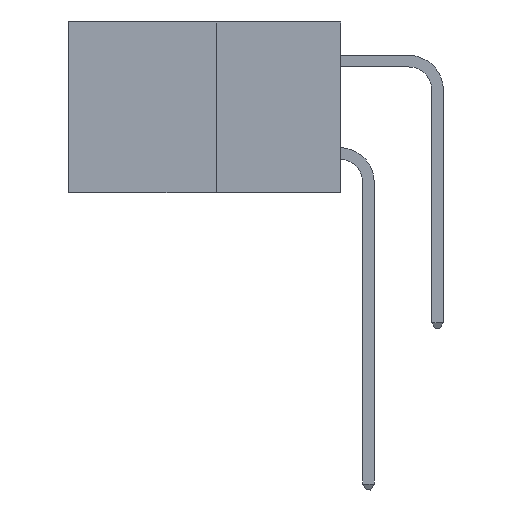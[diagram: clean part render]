
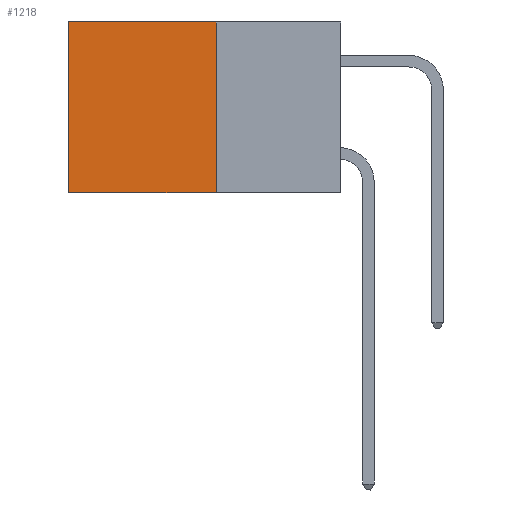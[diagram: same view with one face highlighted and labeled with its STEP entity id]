
A CAD part, left-side view. The second image highlights one B-rep face of the part: STEP entity #1218.
In plain terms, the highlighted planar face has unit normal (-1, 0, 0).
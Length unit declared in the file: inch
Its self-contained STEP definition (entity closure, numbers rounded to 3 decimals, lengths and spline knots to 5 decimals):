
#295 = VERTEX_POINT ( 'NONE', #11340 ) ;
#1195 = DIRECTION ( 'NONE',  ( 0., 0., -1. ) ) ;
#1201 = LINE ( 'NONE', #16741, #13719 ) ;
#1218 = ADVANCED_FACE ( 'NONE', ( #13473 ), #5153, .F. ) ;
#2496 = ORIENTED_EDGE ( 'NONE', *, *, #3451, .T. ) ;
#2753 = DIRECTION ( 'NONE',  ( 1., 0., 0. ) ) ;
#3059 = EDGE_CURVE ( 'NONE', #4408, #295, #4212, .T. ) ;
#3451 = EDGE_CURVE ( 'NONE', #11126, #3791, #7154, .T. ) ;
#3561 = VECTOR ( 'NONE', #5218, 39.37008 ) ;
#3791 = VERTEX_POINT ( 'NONE', #4049 ) ;
#4049 = CARTESIAN_POINT ( 'NONE',  ( 0.277, 0.59, -0.37 ) ) ;
#4212 = LINE ( 'NONE', #13116, #20001 ) ;
#4408 = VERTEX_POINT ( 'NONE', #9347 ) ;
#4413 = CARTESIAN_POINT ( 'NONE',  ( 0.277, 0.59, 0. ) ) ;
#5153 = PLANE ( 'NONE',  #12518 ) ;
#5218 = DIRECTION ( 'NONE',  ( 0., 1., 0. ) ) ;
#5284 = CARTESIAN_POINT ( 'NONE',  ( 0.277, 0.27, 0. ) ) ;
#6318 = CARTESIAN_POINT ( 'NONE',  ( 0.277, 0.59, -0.37 ) ) ;
#6547 = EDGE_CURVE ( 'NONE', #4408, #11126, #7821, .T. ) ;
#7154 = LINE ( 'NONE', #6318, #16928 ) ;
#7260 = ORIENTED_EDGE ( 'NONE', *, *, #18623, .F. ) ;
#7821 = LINE ( 'NONE', #5284, #3561 ) ;
#9347 = CARTESIAN_POINT ( 'NONE',  ( 0.277, 0.27, 0. ) ) ;
#11126 = VERTEX_POINT ( 'NONE', #4413 ) ;
#11340 = CARTESIAN_POINT ( 'NONE',  ( 0.277, 0.27, -0.37 ) ) ;
#12518 = AXIS2_PLACEMENT_3D ( 'NONE', #13528, #2753, #13265 ) ;
#13116 = CARTESIAN_POINT ( 'NONE',  ( 0.277, 0.27, -0.37 ) ) ;
#13265 = DIRECTION ( 'NONE',  ( 0., 0., -1. ) ) ;
#13473 = FACE_OUTER_BOUND ( 'NONE', #16272, .T. ) ;
#13528 = CARTESIAN_POINT ( 'NONE',  ( 0.277, 0.27, -0.37 ) ) ;
#13719 = VECTOR ( 'NONE', #15096, 39.37008 ) ;
#14686 = DIRECTION ( 'NONE',  ( 0., 0., -1. ) ) ;
#15096 = DIRECTION ( 'NONE',  ( 0., 1., 0. ) ) ;
#15977 = ORIENTED_EDGE ( 'NONE', *, *, #3059, .F. ) ;
#16272 = EDGE_LOOP ( 'NONE', ( #2496, #7260, #15977, #20831 ) ) ;
#16741 = CARTESIAN_POINT ( 'NONE',  ( 0.277, 0.27, -0.37 ) ) ;
#16928 = VECTOR ( 'NONE', #1195, 39.37008 ) ;
#18623 = EDGE_CURVE ( 'NONE', #295, #3791, #1201, .T. ) ;
#20001 = VECTOR ( 'NONE', #14686, 39.37008 ) ;
#20831 = ORIENTED_EDGE ( 'NONE', *, *, #6547, .T. ) ;
